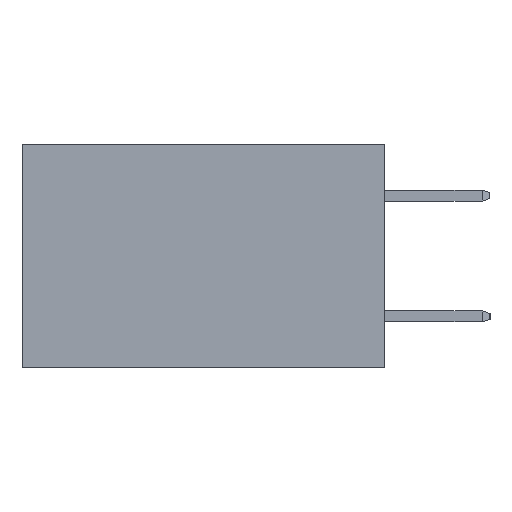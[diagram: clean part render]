
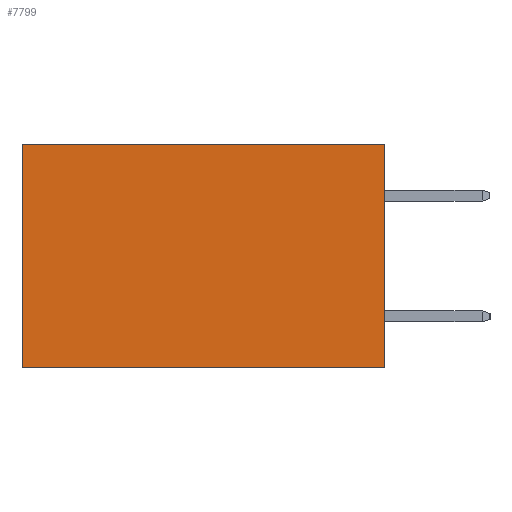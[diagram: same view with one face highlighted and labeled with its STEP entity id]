
A CAD part, left-side view. The second image highlights one B-rep face of the part: STEP entity #7799.
In plain terms, the highlighted planar face has unit normal (-1, 0, 0).
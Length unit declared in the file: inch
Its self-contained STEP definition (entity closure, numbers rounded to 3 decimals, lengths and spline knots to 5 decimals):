
#804 = CARTESIAN_POINT ( 'NONE',  ( 0.2615, 0.6, -0.37 ) ) ;
#902 = EDGE_CURVE ( 'NONE', #8997, #9234, #6159, .T. ) ;
#988 = CARTESIAN_POINT ( 'NONE',  ( 0.2615, 0., -0.37 ) ) ;
#1005 = DIRECTION ( 'NONE',  ( 0., 0., -1. ) ) ;
#1690 = DIRECTION ( 'NONE',  ( 0., 1., 0. ) ) ;
#2319 = LINE ( 'NONE', #6598, #5530 ) ;
#3527 = FACE_OUTER_BOUND ( 'NONE', #5878, .T. ) ;
#3657 = EDGE_CURVE ( 'NONE', #13769, #8997, #2319, .T. ) ;
#3687 = CARTESIAN_POINT ( 'NONE',  ( 0.2615, 0.6, 0. ) ) ;
#4178 = VECTOR ( 'NONE', #1005, 39.37008 ) ;
#4356 = ORIENTED_EDGE ( 'NONE', *, *, #5299, .T. ) ;
#5299 = EDGE_CURVE ( 'NONE', #14611, #9234, #10584, .T. ) ;
#5530 = VECTOR ( 'NONE', #6566, 39.37008 ) ;
#5585 = DIRECTION ( 'NONE',  ( 0., 1., 0. ) ) ;
#5878 = EDGE_LOOP ( 'NONE', ( #4356, #14396, #10420, #9051 ) ) ;
#6159 = LINE ( 'NONE', #6724, #8983 ) ;
#6566 = DIRECTION ( 'NONE',  ( 0., 0., -1. ) ) ;
#6598 = CARTESIAN_POINT ( 'NONE',  ( 0.2615, 0., -0.37 ) ) ;
#6724 = CARTESIAN_POINT ( 'NONE',  ( 0.2615, 0., -0.37 ) ) ;
#7799 = ADVANCED_FACE ( 'NONE', ( #3527 ), #9117, .F. ) ;
#8441 = AXIS2_PLACEMENT_3D ( 'NONE', #9394, #9102, #9087 ) ;
#8445 = LINE ( 'NONE', #12570, #14406 ) ;
#8983 = VECTOR ( 'NONE', #5585, 39.37008 ) ;
#8997 = VERTEX_POINT ( 'NONE', #988 ) ;
#9051 = ORIENTED_EDGE ( 'NONE', *, *, #15316, .T. ) ;
#9087 = DIRECTION ( 'NONE',  ( 0., 0., -1. ) ) ;
#9102 = DIRECTION ( 'NONE',  ( 1., 0., 0. ) ) ;
#9117 = PLANE ( 'NONE',  #8441 ) ;
#9234 = VERTEX_POINT ( 'NONE', #13395 ) ;
#9394 = CARTESIAN_POINT ( 'NONE',  ( 0.2615, 0., -0.37 ) ) ;
#9696 = CARTESIAN_POINT ( 'NONE',  ( 0.2615, 0., 0. ) ) ;
#10420 = ORIENTED_EDGE ( 'NONE', *, *, #3657, .F. ) ;
#10584 = LINE ( 'NONE', #804, #4178 ) ;
#12570 = CARTESIAN_POINT ( 'NONE',  ( 0.2615, 0., 0. ) ) ;
#13395 = CARTESIAN_POINT ( 'NONE',  ( 0.2615, 0.6, -0.37 ) ) ;
#13769 = VERTEX_POINT ( 'NONE', #9696 ) ;
#14396 = ORIENTED_EDGE ( 'NONE', *, *, #902, .F. ) ;
#14406 = VECTOR ( 'NONE', #1690, 39.37008 ) ;
#14611 = VERTEX_POINT ( 'NONE', #3687 ) ;
#15316 = EDGE_CURVE ( 'NONE', #13769, #14611, #8445, .T. ) ;
